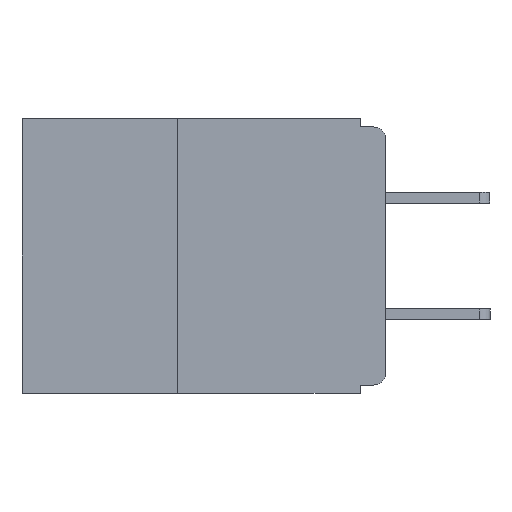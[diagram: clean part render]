
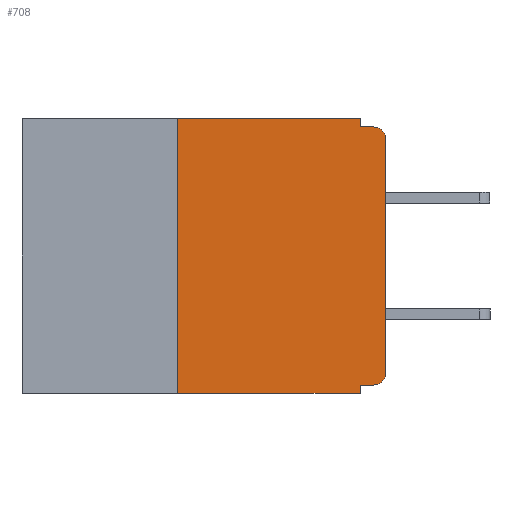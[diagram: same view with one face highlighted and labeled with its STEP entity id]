
A CAD part, left-side view. The second image highlights one B-rep face of the part: STEP entity #708.
In plain terms, the highlighted planar face has unit normal (-1, 0, 0).
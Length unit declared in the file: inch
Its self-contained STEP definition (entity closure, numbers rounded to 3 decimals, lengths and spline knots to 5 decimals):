
#283 = DIRECTION ( 'NONE',  ( -1., 0., 0. ) ) ;
#295 = ORIENTED_EDGE ( 'NONE', *, *, #9227, .F. ) ;
#708 = ADVANCED_FACE ( 'NONE', ( #27367 ), #14077, .F. ) ;
#1049 = DIRECTION ( 'NONE',  ( 0., -1., 0. ) ) ;
#1303 = EDGE_CURVE ( 'NONE', #7804, #17327, #10230, .T. ) ;
#1552 = DIRECTION ( 'NONE',  ( 0., 0., -1. ) ) ;
#1580 = LINE ( 'NONE', #22395, #13292 ) ;
#2441 = LINE ( 'NONE', #12648, #15598 ) ;
#2618 = CARTESIAN_POINT ( 'NONE',  ( 0., 0.437, -0.33 ) ) ;
#3173 = CARTESIAN_POINT ( 'NONE',  ( 0., 0.015, -0.305 ) ) ;
#3398 = CARTESIAN_POINT ( 'NONE',  ( 0., 0.031, -0.33 ) ) ;
#3474 = DIRECTION ( 'NONE',  ( 0., 0., 1. ) ) ;
#4863 = VERTEX_POINT ( 'NONE', #15093 ) ;
#4882 = DIRECTION ( 'NONE',  ( 0., 0., -1. ) ) ;
#5014 = DIRECTION ( 'NONE',  ( 0., -1., 0. ) ) ;
#5573 = DIRECTION ( 'NONE',  ( 0., 0., -1. ) ) ;
#5698 = VERTEX_POINT ( 'NONE', #3398 ) ;
#7755 = VERTEX_POINT ( 'NONE', #22676 ) ;
#7804 = VERTEX_POINT ( 'NONE', #27416 ) ;
#8002 = EDGE_CURVE ( 'NONE', #7755, #5698, #16191, .T. ) ;
#8042 = LINE ( 'NONE', #17382, #26995 ) ;
#8727 = DIRECTION ( 'NONE',  ( 0., 1., 0. ) ) ;
#9168 = DIRECTION ( 'NONE',  ( 1., 0., 0. ) ) ;
#9227 = EDGE_CURVE ( 'NONE', #17449, #7755, #1580, .T. ) ;
#9596 = VERTEX_POINT ( 'NONE', #19183 ) ;
#10230 = CIRCLE ( 'NONE', #29070, 0.015 ) ;
#11454 = CARTESIAN_POINT ( 'NONE',  ( 0., 0.437, 0. ) ) ;
#11905 = VECTOR ( 'NONE', #13013, 39.37008 ) ;
#12179 = CARTESIAN_POINT ( 'NONE',  ( 0., 0.031, -0.33 ) ) ;
#12618 = VECTOR ( 'NONE', #27360, 39.37008 ) ;
#12648 = CARTESIAN_POINT ( 'NONE',  ( 0., 0.031, 0. ) ) ;
#12958 = AXIS2_PLACEMENT_3D ( 'NONE', #14073, #9168, #1552 ) ;
#13013 = DIRECTION ( 'NONE',  ( 0., 0., 1. ) ) ;
#13117 = VERTEX_POINT ( 'NONE', #28281 ) ;
#13274 = EDGE_CURVE ( 'NONE', #19462, #7804, #14065, .T. ) ;
#13292 = VECTOR ( 'NONE', #8727, 39.37008 ) ;
#13431 = LINE ( 'NONE', #15035, #24874 ) ;
#13447 = ORIENTED_EDGE ( 'NONE', *, *, #24569, .F. ) ;
#13794 = ORIENTED_EDGE ( 'NONE', *, *, #1303, .T. ) ;
#14065 = LINE ( 'NONE', #15327, #11905 ) ;
#14073 = CARTESIAN_POINT ( 'NONE',  ( 0., 0.437, 0. ) ) ;
#14077 = PLANE ( 'NONE',  #12958 ) ;
#14199 = EDGE_CURVE ( 'NONE', #13117, #5698, #27836, .T. ) ;
#14510 = DIRECTION ( 'NONE',  ( 0., 0., -1. ) ) ;
#14582 = EDGE_LOOP ( 'NONE', ( #24524, #13794, #13447, #17037, #21296, #16696, #28693, #18117, #295, #19541 ) ) ;
#15035 = CARTESIAN_POINT ( 'NONE',  ( 0., 0., -0.01 ) ) ;
#15093 = CARTESIAN_POINT ( 'NONE',  ( 0., 0.031, 0. ) ) ;
#15238 = AXIS2_PLACEMENT_3D ( 'NONE', #3173, #19356, #5573 ) ;
#15327 = CARTESIAN_POINT ( 'NONE',  ( 0., 0., 0. ) ) ;
#15598 = VECTOR ( 'NONE', #28507, 39.37008 ) ;
#16096 = VERTEX_POINT ( 'NONE', #24125 ) ;
#16191 = LINE ( 'NONE', #12179, #27529 ) ;
#16696 = ORIENTED_EDGE ( 'NONE', *, *, #23354, .F. ) ;
#17037 = ORIENTED_EDGE ( 'NONE', *, *, #27870, .F. ) ;
#17264 = CARTESIAN_POINT ( 'NONE',  ( 0., 0., -0.305 ) ) ;
#17327 = VERTEX_POINT ( 'NONE', #28432 ) ;
#17382 = CARTESIAN_POINT ( 'NONE',  ( 0., 0.25, -0.33 ) ) ;
#17449 = VERTEX_POINT ( 'NONE', #19764 ) ;
#18117 = ORIENTED_EDGE ( 'NONE', *, *, #8002, .F. ) ;
#19183 = CARTESIAN_POINT ( 'NONE',  ( 0., 0.031, -0.01 ) ) ;
#19356 = DIRECTION ( 'NONE',  ( -1., 0., 0. ) ) ;
#19462 = VERTEX_POINT ( 'NONE', #17264 ) ;
#19541 = ORIENTED_EDGE ( 'NONE', *, *, #25134, .T. ) ;
#19764 = CARTESIAN_POINT ( 'NONE',  ( 0., 0.015, -0.32 ) ) ;
#19818 = EDGE_CURVE ( 'NONE', #16096, #4863, #24042, .T. ) ;
#21296 = ORIENTED_EDGE ( 'NONE', *, *, #19818, .F. ) ;
#22395 = CARTESIAN_POINT ( 'NONE',  ( 0., 0., -0.32 ) ) ;
#22544 = VECTOR ( 'NONE', #5014, 39.37008 ) ;
#22676 = CARTESIAN_POINT ( 'NONE',  ( 0., 0.031, -0.32 ) ) ;
#23354 = EDGE_CURVE ( 'NONE', #13117, #16096, #8042, .T. ) ;
#23594 = CARTESIAN_POINT ( 'NONE',  ( 0., 0.015, -0.025 ) ) ;
#24042 = LINE ( 'NONE', #11454, #12618 ) ;
#24125 = CARTESIAN_POINT ( 'NONE',  ( 0., 0.25, 0. ) ) ;
#24524 = ORIENTED_EDGE ( 'NONE', *, *, #13274, .T. ) ;
#24569 = EDGE_CURVE ( 'NONE', #9596, #17327, #13431, .T. ) ;
#24874 = VECTOR ( 'NONE', #1049, 39.37008 ) ;
#25134 = EDGE_CURVE ( 'NONE', #17449, #19462, #26114, .T. ) ;
#26114 = CIRCLE ( 'NONE', #15238, 0.015 ) ;
#26995 = VECTOR ( 'NONE', #3474, 39.37008 ) ;
#27360 = DIRECTION ( 'NONE',  ( 0., -1., 0. ) ) ;
#27367 = FACE_OUTER_BOUND ( 'NONE', #14582, .T. ) ;
#27416 = CARTESIAN_POINT ( 'NONE',  ( 0., 0., -0.025 ) ) ;
#27529 = VECTOR ( 'NONE', #14510, 39.37008 ) ;
#27836 = LINE ( 'NONE', #2618, #22544 ) ;
#27870 = EDGE_CURVE ( 'NONE', #4863, #9596, #2441, .T. ) ;
#28281 = CARTESIAN_POINT ( 'NONE',  ( 0., 0.25, -0.33 ) ) ;
#28432 = CARTESIAN_POINT ( 'NONE',  ( 0., 0.015, -0.01 ) ) ;
#28507 = DIRECTION ( 'NONE',  ( 0., 0., -1. ) ) ;
#28693 = ORIENTED_EDGE ( 'NONE', *, *, #14199, .T. ) ;
#29070 = AXIS2_PLACEMENT_3D ( 'NONE', #23594, #283, #4882 ) ;
